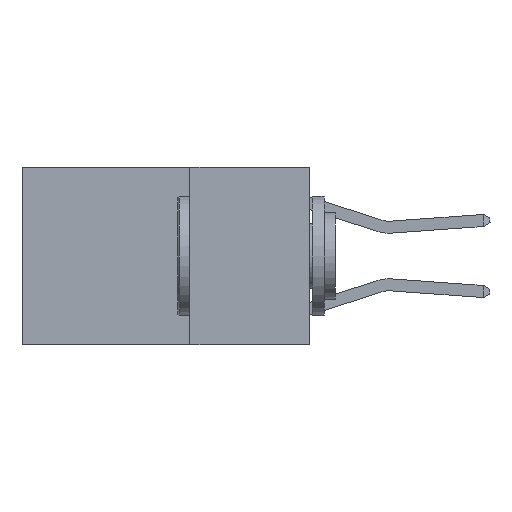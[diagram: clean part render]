
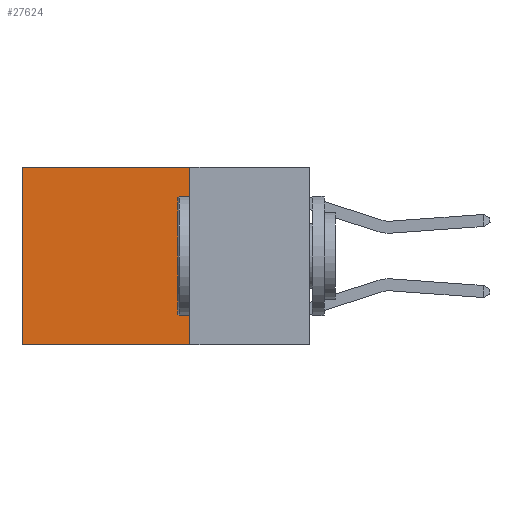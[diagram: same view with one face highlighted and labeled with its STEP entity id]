
A CAD part, left-side view. The second image highlights one B-rep face of the part: STEP entity #27624.
In plain terms, the highlighted planar face has unit normal (-1, 0, 0).
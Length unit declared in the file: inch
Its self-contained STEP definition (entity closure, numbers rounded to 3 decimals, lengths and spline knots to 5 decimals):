
#1417 = ORIENTED_EDGE ( 'NONE', *, *, #6398, .F. ) ;
#2806 = VECTOR ( 'NONE', #13541, 39.37008 ) ;
#4265 = CARTESIAN_POINT ( 'NONE',  ( 0.2625, 0.6, 0. ) ) ;
#5981 = PLANE ( 'NONE',  #7721 ) ;
#6068 = EDGE_CURVE ( 'NONE', #26363, #25826, #30256, .T. ) ;
#6398 = EDGE_CURVE ( 'NONE', #22555, #26363, #18513, .T. ) ;
#7045 = CARTESIAN_POINT ( 'NONE',  ( 0.2625, 0.25, 0. ) ) ;
#7607 = EDGE_LOOP ( 'NONE', ( #29347, #14401, #1417, #24886 ) ) ;
#7721 = AXIS2_PLACEMENT_3D ( 'NONE', #25416, #15639, #20983 ) ;
#9160 = DIRECTION ( 'NONE',  ( 0., 0., -1. ) ) ;
#9714 = VECTOR ( 'NONE', #18506, 39.37008 ) ;
#10908 = VECTOR ( 'NONE', #9160, 39.37008 ) ;
#11229 = LINE ( 'NONE', #20863, #9714 ) ;
#11929 = VECTOR ( 'NONE', #29073, 39.37008 ) ;
#13541 = DIRECTION ( 'NONE',  ( 0., 1., 0. ) ) ;
#14401 = ORIENTED_EDGE ( 'NONE', *, *, #6068, .F. ) ;
#15600 = CARTESIAN_POINT ( 'NONE',  ( 0.2625, 0.25, -0.37 ) ) ;
#15639 = DIRECTION ( 'NONE',  ( 1., 0., 0. ) ) ;
#18506 = DIRECTION ( 'NONE',  ( 0., 0., -1. ) ) ;
#18513 = LINE ( 'NONE', #28135, #10908 ) ;
#20863 = CARTESIAN_POINT ( 'NONE',  ( 0.2625, 0.6, 0. ) ) ;
#20983 = DIRECTION ( 'NONE',  ( 0., 0., -1. ) ) ;
#21552 = EDGE_CURVE ( 'NONE', #22555, #27147, #26243, .T. ) ;
#22555 = VERTEX_POINT ( 'NONE', #7045 ) ;
#23347 = CARTESIAN_POINT ( 'NONE',  ( 0.2625, 0.6, -0.37 ) ) ;
#24547 = CARTESIAN_POINT ( 'NONE',  ( 0.2625, 0.25, -0.37 ) ) ;
#24886 = ORIENTED_EDGE ( 'NONE', *, *, #21552, .T. ) ;
#25416 = CARTESIAN_POINT ( 'NONE',  ( 0.2625, 0.25, 0. ) ) ;
#25826 = VERTEX_POINT ( 'NONE', #23347 ) ;
#26243 = LINE ( 'NONE', #28605, #11929 ) ;
#26363 = VERTEX_POINT ( 'NONE', #24547 ) ;
#27147 = VERTEX_POINT ( 'NONE', #4265 ) ;
#27231 = EDGE_CURVE ( 'NONE', #27147, #25826, #11229, .T. ) ;
#27624 = ADVANCED_FACE ( 'NONE', ( #29994 ), #5981, .F. ) ;
#28135 = CARTESIAN_POINT ( 'NONE',  ( 0.2625, 0.25, 0. ) ) ;
#28605 = CARTESIAN_POINT ( 'NONE',  ( 0.2625, 0.25, 0. ) ) ;
#29073 = DIRECTION ( 'NONE',  ( 0., 1., 0. ) ) ;
#29347 = ORIENTED_EDGE ( 'NONE', *, *, #27231, .T. ) ;
#29994 = FACE_OUTER_BOUND ( 'NONE', #7607, .T. ) ;
#30256 = LINE ( 'NONE', #15600, #2806 ) ;
